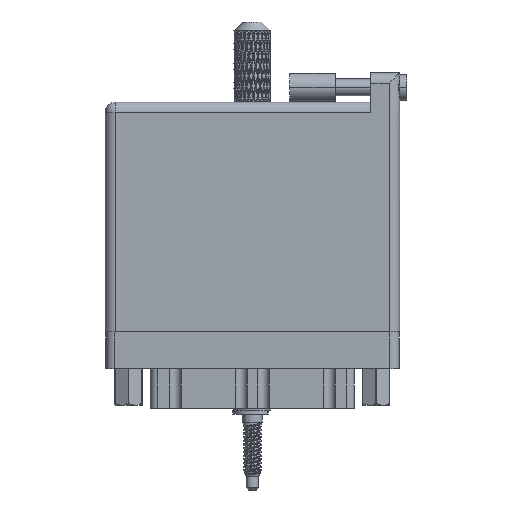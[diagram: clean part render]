
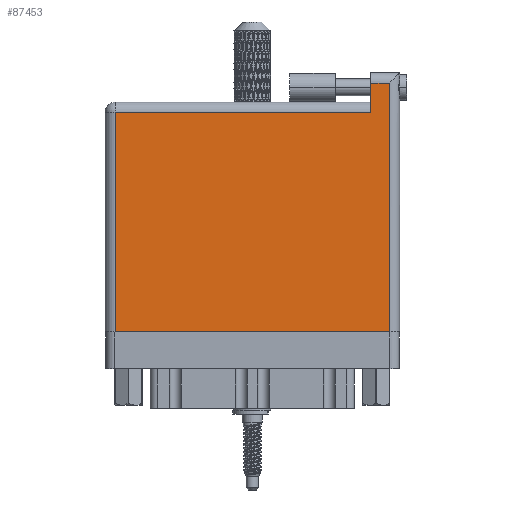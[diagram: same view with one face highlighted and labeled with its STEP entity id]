
A CAD part, front view. The second image highlights one B-rep face of the part: STEP entity #87453.
In plain terms, the highlighted face is planar.
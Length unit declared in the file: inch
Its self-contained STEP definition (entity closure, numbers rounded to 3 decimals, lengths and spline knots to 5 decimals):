
#6049 = VECTOR ( 'NONE', #45952, 39.37008 ) ;
#11600 = ORIENTED_EDGE ( 'NONE', *, *, #100703, .T. ) ;
#11934 = ORIENTED_EDGE ( 'NONE', *, *, #15443, .T. ) ;
#14062 = CARTESIAN_POINT ( 'NONE',  ( 0., 1.696, 0. ) ) ;
#15443 = EDGE_CURVE ( 'NONE', #66015, #85860, #49678, .T. ) ;
#19135 = CARTESIAN_POINT ( 'NONE',  ( 0.07, 0., 0. ) ) ;
#21549 = VERTEX_POINT ( 'NONE', #51037 ) ;
#22311 = CARTESIAN_POINT ( 'NONE',  ( 0.07, 0., 0. ) ) ;
#23382 = DIRECTION ( 'NONE',  ( -1., 0., 0. ) ) ;
#26216 = EDGE_CURVE ( 'NONE', #105856, #21549, #83370, .T. ) ;
#26270 = FACE_OUTER_BOUND ( 'NONE', #87625, .T. ) ;
#26886 = CARTESIAN_POINT ( 'NONE',  ( 1.811, 1.496, 0. ) ) ;
#30619 = LINE ( 'NONE', #14062, #91005 ) ;
#32022 = AXIS2_PLACEMENT_3D ( 'NONE', #111969, #52576, #70235 ) ;
#32794 = VERTEX_POINT ( 'NONE', #35376 ) ;
#34299 = LINE ( 'NONE', #96551, #53051 ) ;
#35376 = CARTESIAN_POINT ( 'NONE',  ( 1.811, 1.696, 0. ) ) ;
#36239 = LINE ( 'NONE', #62500, #6049 ) ;
#36567 = DIRECTION ( 'NONE',  ( 1., 0., 0. ) ) ;
#40011 = LINE ( 'NONE', #22311, #51862 ) ;
#40525 = CARTESIAN_POINT ( 'NONE',  ( 0., 1.496, 0. ) ) ;
#44164 = EDGE_CURVE ( 'NONE', #32794, #66015, #36239, .T. ) ;
#45952 = DIRECTION ( 'NONE',  ( 0., -1., 0. ) ) ;
#46674 = CARTESIAN_POINT ( 'NONE',  ( 1.938, 0., 0. ) ) ;
#47993 = DIRECTION ( 'NONE',  ( 0., 1., 0. ) ) ;
#48986 = EDGE_CURVE ( 'NONE', #21549, #32794, #30619, .T. ) ;
#49678 = LINE ( 'NONE', #40525, #102567 ) ;
#51037 = CARTESIAN_POINT ( 'NONE',  ( 1.938, 1.696, 0. ) ) ;
#51862 = VECTOR ( 'NONE', #85095, 39.37008 ) ;
#52576 = DIRECTION ( 'NONE',  ( 0., 0., -1. ) ) ;
#53051 = VECTOR ( 'NONE', #36567, 39.37008 ) ;
#58406 = ORIENTED_EDGE ( 'NONE', *, *, #48986, .T. ) ;
#62500 = CARTESIAN_POINT ( 'NONE',  ( 1.811, 1.766, 0. ) ) ;
#66015 = VERTEX_POINT ( 'NONE', #26886 ) ;
#66038 = EDGE_CURVE ( 'NONE', #112591, #105856, #34299, .T. ) ;
#68148 = ORIENTED_EDGE ( 'NONE', *, *, #44164, .T. ) ;
#70235 = DIRECTION ( 'NONE',  ( -1., 0., 0. ) ) ;
#76425 = ORIENTED_EDGE ( 'NONE', *, *, #66038, .T. ) ;
#77601 = VECTOR ( 'NONE', #47993, 39.37008 ) ;
#81133 = CARTESIAN_POINT ( 'NONE',  ( 1.938, 1.766, 0. ) ) ;
#83370 = LINE ( 'NONE', #81133, #77601 ) ;
#85095 = DIRECTION ( 'NONE',  ( 0., -1., 0. ) ) ;
#85386 = DIRECTION ( 'NONE',  ( -1., 0., 0. ) ) ;
#85860 = VERTEX_POINT ( 'NONE', #86186 ) ;
#86186 = CARTESIAN_POINT ( 'NONE',  ( 0.07, 1.496, 0. ) ) ;
#86834 = PLANE ( 'NONE',  #32022 ) ;
#87453 = ADVANCED_FACE ( 'NONE', ( #26270 ), #86834, .F. ) ;
#87625 = EDGE_LOOP ( 'NONE', ( #76425, #106561, #58406, #68148, #11934, #11600 ) ) ;
#91005 = VECTOR ( 'NONE', #85386, 39.37008 ) ;
#96551 = CARTESIAN_POINT ( 'NONE',  ( 0., 0., 0. ) ) ;
#100703 = EDGE_CURVE ( 'NONE', #85860, #112591, #40011, .T. ) ;
#102567 = VECTOR ( 'NONE', #23382, 39.37008 ) ;
#105856 = VERTEX_POINT ( 'NONE', #46674 ) ;
#106561 = ORIENTED_EDGE ( 'NONE', *, *, #26216, .T. ) ;
#111969 = CARTESIAN_POINT ( 'NONE',  ( 0., 1.566, 0. ) ) ;
#112591 = VERTEX_POINT ( 'NONE', #19135 ) ;
